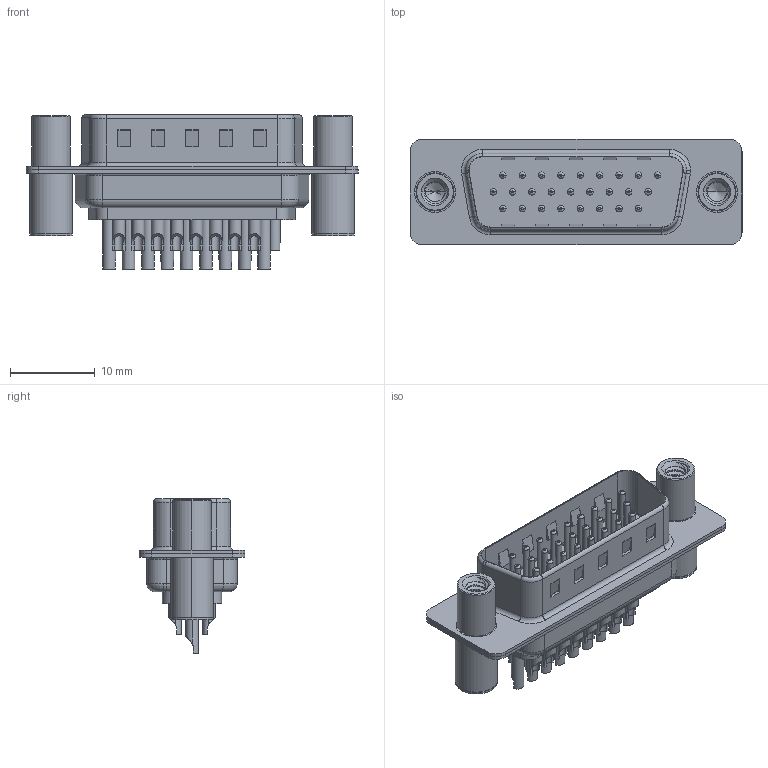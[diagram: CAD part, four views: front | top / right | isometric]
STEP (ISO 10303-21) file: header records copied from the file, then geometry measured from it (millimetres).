
FILE_DESCRIPTION (( 'STEP AP203' ), '1' );
FILE_NAME ('637-M26-332-BN4.STEP', '2018-11-19T23:51:54', ( '' ), ( '' ), 'SwSTEP 2.0', 'SolidWorks 2016', '' );
FILE_SCHEMA (( 'CONFIG_CONTROL_DESIGN' ));
Length unit declared in the file: millimetre
Products named in the file (8): 637M Contact Row 2_32; 637M Contact Row 3_32; 637M 4-40 Threaded Standoff and Board Spacer; 637-M26-332-BN4; 637M Housing_26 Contacts; 637M Shell Front_26 Contacts; 637M Shell Rear_26 Contacts; 637M Contact Row 1_32
Assembly tree (31 placements, depth 2):
  637-M26-332-BN4
    637M Housing_26 Contacts
    637M Shell Front_26 Contacts
    637M Shell Rear_26 Contacts
    637M Contact Row 1_32  x9
    637M Contact Row 2_32  x9
    637M Contact Row 3_32  x8
    637M 4-40 Threaded Standoff and Board Spacer  x2
Bounding box: 39.2 x 12.5 x 18.25 mm (x, y, z)
Volume: 2282.7 mm3; surface area: 6602.4 mm2
Topology: 31 solids, 31 shells, 1388 faces, 3267 edges, 2002 vertices
Faces by surface type: cylinder 601, plane 379, torus 314, cone 82, bspline 12
Entity records: 22662 total; most frequent: CARTESIAN_POINT 5615, DIRECTION 3474, ORIENTED_EDGE 3090, EDGE_CURVE 1545, AXIS2_PLACEMENT_3D 1386, VERTEX_POINT 984, EDGE_LOOP 799, CIRCLE 713
